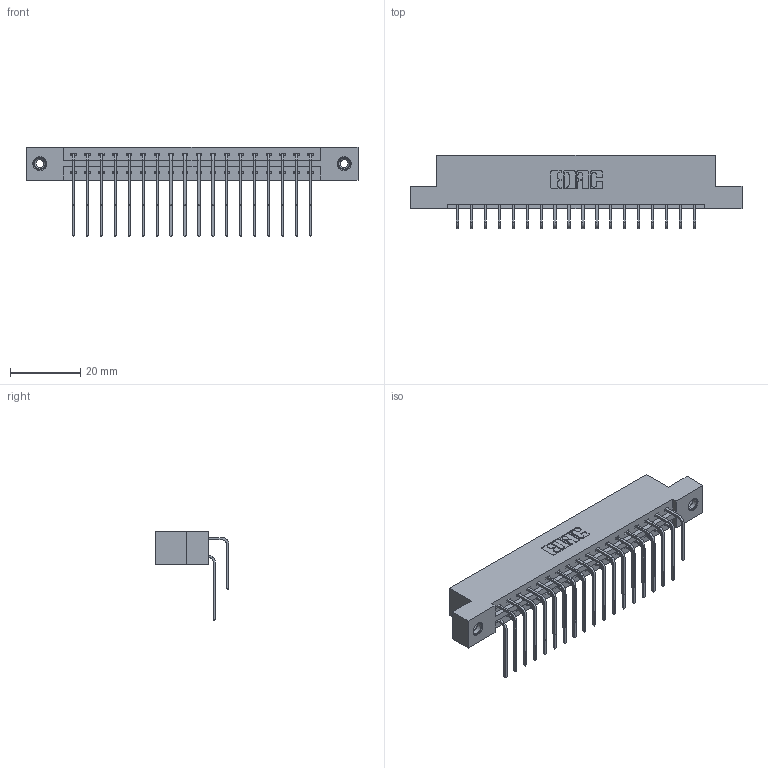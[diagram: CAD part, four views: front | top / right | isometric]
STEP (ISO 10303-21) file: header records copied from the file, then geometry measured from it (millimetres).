
FILE_DESCRIPTION (( 'STEP AP203' ), '1' );
FILE_NAME ('387-036-559-208.STEP', '2019-10-17T20:20:29', ( '' ), ( '' ), 'SwSTEP 2.0', 'SolidWorks 2016', '' );
FILE_SCHEMA (( 'CONFIG_CONTROL_DESIGN' ));
Length unit declared in the file: inch
Products named in the file (5): 337 Part_Flush Mounting Lugs - 0.156 Dia-TI; 345-250-001_345-250-003-102; 345-292-001_559 Tail - 2; 345-292-001_558 559 Tail - 1; 387-036-559-208
Assembly tree (39 placements, depth 2):
  387-036-559-208
    337 Part_Flush Mounting Lugs - 0.156 Dia-TI
    345-292-001_558 559 Tail - 1  x18
    345-292-001_559 Tail - 2  x18
    345-250-001_345-250-003-102  x2
Bounding box: 94.34 x 20.9 x 25.53 mm (x, y, z)
Volume: 9823.5 mm3; surface area: 11939.1 mm2
Topology: 39 solids, 39 shells, 2190 faces, 6459 edges, 4250 vertices
Faces by surface type: plane 1542, cylinder 632, cone 12, torus 4
Entity records: 20030 total; most frequent: CARTESIAN_POINT 3420, ORIENTED_EDGE 3298, DIRECTION 2967, EDGE_CURVE 1649, LINE 1461, VECTOR 1461, VERTEX_POINT 1092, AXIS2_PLACEMENT_3D 753
